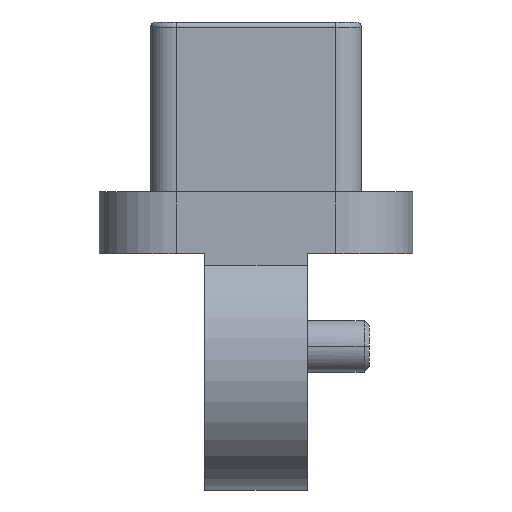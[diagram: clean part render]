
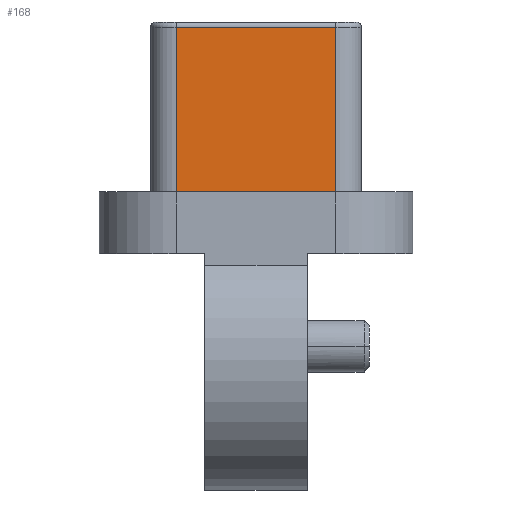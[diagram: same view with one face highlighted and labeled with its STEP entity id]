
A CAD part, left-side view. The second image highlights one B-rep face of the part: STEP entity #168.
In plain terms, the highlighted planar face has unit normal (-1, 0, 0).
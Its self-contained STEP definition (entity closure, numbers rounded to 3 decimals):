
#44 = CARTESIAN_POINT ( 'NONE',  ( -9.65, -1.55, -3.3 ) ) ;
#168 = ADVANCED_FACE ( 'NONE', ( #1551 ), #4044, .F. ) ;
#393 = VERTEX_POINT ( 'NONE', #615 ) ;
#542 = LINE ( 'NONE', #3013, #3977 ) ;
#615 = CARTESIAN_POINT ( 'NONE',  ( -9.65, -1.55, -0.1 ) ) ;
#625 = CARTESIAN_POINT ( 'NONE',  ( -9.65, -1.55, -0.1 ) ) ;
#941 = DIRECTION ( 'NONE',  ( 1., 0., 0. ) ) ;
#1551 = FACE_OUTER_BOUND ( 'NONE', #2601, .T. ) ;
#1690 = CARTESIAN_POINT ( 'NONE',  ( -9.65, -1.55, -3.3 ) ) ;
#2223 = VECTOR ( 'NONE', #3100, 1000. ) ;
#2252 = AXIS2_PLACEMENT_3D ( 'NONE', #6527, #941, #3429 ) ;
#2365 = CARTESIAN_POINT ( 'NONE',  ( -9.65, 1.55, -0.1 ) ) ;
#2601 = EDGE_LOOP ( 'NONE', ( #5053, #7083, #5787, #4149 ) ) ;
#2780 = EDGE_CURVE ( 'NONE', #3707, #7989, #2877, .T. ) ;
#2877 = LINE ( 'NONE', #5369, #6359 ) ;
#3013 = CARTESIAN_POINT ( 'NONE',  ( -9.65, 1.55, -3.3 ) ) ;
#3100 = DIRECTION ( 'NONE',  ( 0., 1., 0. ) ) ;
#3429 = DIRECTION ( 'NONE',  ( 0., 1., 0. ) ) ;
#3707 = VERTEX_POINT ( 'NONE', #2365 ) ;
#3977 = VECTOR ( 'NONE', #5515, 1000. ) ;
#4044 = PLANE ( 'NONE',  #2252 ) ;
#4108 = VERTEX_POINT ( 'NONE', #44 ) ;
#4149 = ORIENTED_EDGE ( 'NONE', *, *, #4949, .T. ) ;
#4181 = DIRECTION ( 'NONE',  ( 0., 0., 1. ) ) ;
#4624 = VECTOR ( 'NONE', #4181, 1000. ) ;
#4949 = EDGE_CURVE ( 'NONE', #393, #3707, #6205, .T. ) ;
#5053 = ORIENTED_EDGE ( 'NONE', *, *, #2780, .T. ) ;
#5369 = CARTESIAN_POINT ( 'NONE',  ( -9.65, 1.55, -0.1 ) ) ;
#5498 = CARTESIAN_POINT ( 'NONE',  ( -9.65, 1.55, -3.3 ) ) ;
#5515 = DIRECTION ( 'NONE',  ( 0., -1., 0. ) ) ;
#5787 = ORIENTED_EDGE ( 'NONE', *, *, #6317, .T. ) ;
#6205 = LINE ( 'NONE', #625, #2223 ) ;
#6317 = EDGE_CURVE ( 'NONE', #4108, #393, #7294, .T. ) ;
#6359 = VECTOR ( 'NONE', #7859, 1000. ) ;
#6527 = CARTESIAN_POINT ( 'NONE',  ( -9.65, 0., -1.7 ) ) ;
#6677 = EDGE_CURVE ( 'NONE', #7989, #4108, #542, .T. ) ;
#7083 = ORIENTED_EDGE ( 'NONE', *, *, #6677, .T. ) ;
#7294 = LINE ( 'NONE', #1690, #4624 ) ;
#7859 = DIRECTION ( 'NONE',  ( 0., 0., -1. ) ) ;
#7989 = VERTEX_POINT ( 'NONE', #5498 ) ;
